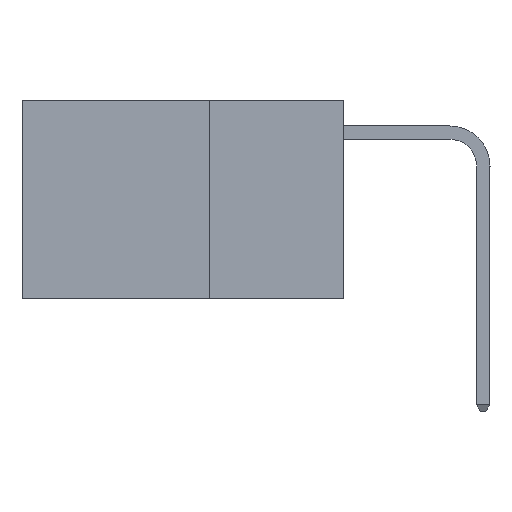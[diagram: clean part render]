
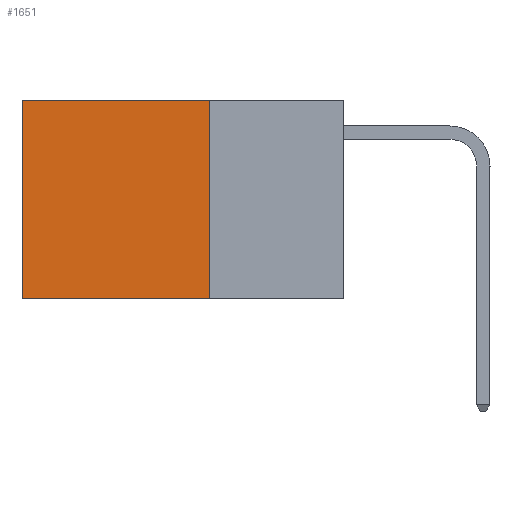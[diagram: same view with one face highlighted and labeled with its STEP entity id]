
A CAD part, left-side view. The second image highlights one B-rep face of the part: STEP entity #1651.
In plain terms, the highlighted planar face has unit normal (-1, 0, 0).
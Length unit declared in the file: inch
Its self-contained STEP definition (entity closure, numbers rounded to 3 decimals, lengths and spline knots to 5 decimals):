
#358 = VECTOR ( 'NONE', #1797, 39.37008 ) ;
#542 = CARTESIAN_POINT ( 'NONE',  ( 0.2625, 0.25, 0. ) ) ;
#807 = CARTESIAN_POINT ( 'NONE',  ( 0.2625, 0.6, 0. ) ) ;
#864 = ORIENTED_EDGE ( 'NONE', *, *, #9592, .T. ) ;
#941 = VERTEX_POINT ( 'NONE', #807 ) ;
#1534 = DIRECTION ( 'NONE',  ( 0., 1., 0. ) ) ;
#1604 = VERTEX_POINT ( 'NONE', #3416 ) ;
#1651 = ADVANCED_FACE ( 'NONE', ( #10301 ), #7094, .F. ) ;
#1717 = DIRECTION ( 'NONE',  ( 0., 0., -1. ) ) ;
#1797 = DIRECTION ( 'NONE',  ( 0., 0., -1. ) ) ;
#2575 = DIRECTION ( 'NONE',  ( 0., 0., -1. ) ) ;
#2724 = LINE ( 'NONE', #8629, #358 ) ;
#2921 = CARTESIAN_POINT ( 'NONE',  ( 0.2625, 0.25, -0.37 ) ) ;
#2927 = EDGE_CURVE ( 'NONE', #1604, #4511, #2724, .T. ) ;
#3416 = CARTESIAN_POINT ( 'NONE',  ( 0.2625, 0.25, 0. ) ) ;
#3485 = EDGE_LOOP ( 'NONE', ( #864, #6162, #7497, #6742 ) ) ;
#4511 = VERTEX_POINT ( 'NONE', #2921 ) ;
#4632 = VECTOR ( 'NONE', #1534, 39.37008 ) ;
#4872 = DIRECTION ( 'NONE',  ( 0., 1., 0. ) ) ;
#5897 = VERTEX_POINT ( 'NONE', #7207 ) ;
#6162 = ORIENTED_EDGE ( 'NONE', *, *, #10779, .F. ) ;
#6742 = ORIENTED_EDGE ( 'NONE', *, *, #7807, .T. ) ;
#7094 = PLANE ( 'NONE',  #12277 ) ;
#7207 = CARTESIAN_POINT ( 'NONE',  ( 0.2625, 0.6, -0.37 ) ) ;
#7411 = DIRECTION ( 'NONE',  ( 1., 0., 0. ) ) ;
#7497 = ORIENTED_EDGE ( 'NONE', *, *, #2927, .F. ) ;
#7599 = CARTESIAN_POINT ( 'NONE',  ( 0.2625, 0.25, 0. ) ) ;
#7784 = VECTOR ( 'NONE', #4872, 39.37008 ) ;
#7807 = EDGE_CURVE ( 'NONE', #1604, #941, #9736, .T. ) ;
#8629 = CARTESIAN_POINT ( 'NONE',  ( 0.2625, 0.25, 0. ) ) ;
#9143 = VECTOR ( 'NONE', #2575, 39.37008 ) ;
#9455 = LINE ( 'NONE', #12141, #9143 ) ;
#9592 = EDGE_CURVE ( 'NONE', #941, #5897, #9455, .T. ) ;
#9736 = LINE ( 'NONE', #542, #4632 ) ;
#10031 = LINE ( 'NONE', #10614, #7784 ) ;
#10301 = FACE_OUTER_BOUND ( 'NONE', #3485, .T. ) ;
#10614 = CARTESIAN_POINT ( 'NONE',  ( 0.2625, 0.25, -0.37 ) ) ;
#10779 = EDGE_CURVE ( 'NONE', #4511, #5897, #10031, .T. ) ;
#12141 = CARTESIAN_POINT ( 'NONE',  ( 0.2625, 0.6, 0. ) ) ;
#12277 = AXIS2_PLACEMENT_3D ( 'NONE', #7599, #7411, #1717 ) ;
